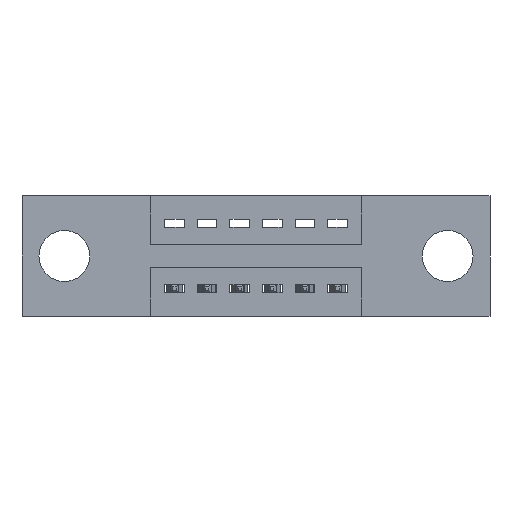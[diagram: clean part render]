
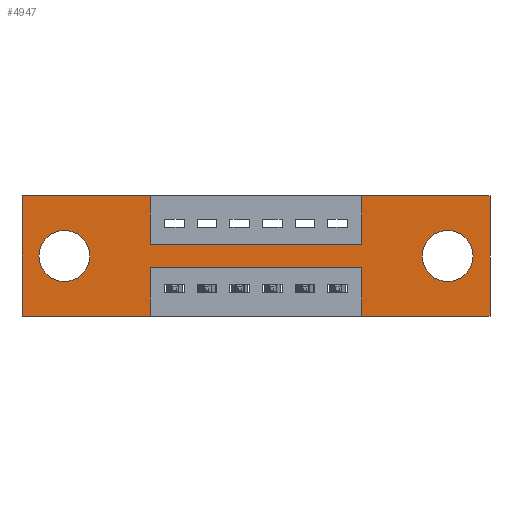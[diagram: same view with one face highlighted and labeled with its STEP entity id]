
A CAD part, front view. The second image highlights one B-rep face of the part: STEP entity #4947.
In plain terms, the highlighted planar face has unit normal (0, -1, 0).
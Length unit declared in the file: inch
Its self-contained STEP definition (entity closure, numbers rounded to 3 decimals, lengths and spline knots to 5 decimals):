
#31 = ORIENTED_EDGE ( 'NONE', *, *, #5997, .F. ) ;
#70 = ORIENTED_EDGE ( 'NONE', *, *, #4666, .F. ) ;
#135 = VECTOR ( 'NONE', #2816, 39.37008 ) ;
#189 = DIRECTION ( 'NONE',  ( 0., 0., -1. ) ) ;
#243 = FACE_BOUND ( 'NONE', #8866, .T. ) ;
#315 = DIRECTION ( 'NONE',  ( 0., 1., 0. ) ) ;
#382 = CARTESIAN_POINT ( 'NONE',  ( 0.13, 0., -0.185 ) ) ;
#444 = AXIS2_PLACEMENT_3D ( 'NONE', #957, #8113, #189 ) ;
#468 = PLANE ( 'NONE',  #444 ) ;
#481 = LINE ( 'NONE', #1972, #6786 ) ;
#488 = CARTESIAN_POINT ( 'NONE',  ( 0.13, 0., -0.263 ) ) ;
#525 = DIRECTION ( 'NONE',  ( 1., 0., 0. ) ) ;
#559 = ORIENTED_EDGE ( 'NONE', *, *, #8038, .F. ) ;
#597 = ORIENTED_EDGE ( 'NONE', *, *, #9324, .F. ) ;
#759 = CARTESIAN_POINT ( 'NONE',  ( 0., 0., 0. ) ) ;
#957 = CARTESIAN_POINT ( 'NONE',  ( 0., 0., -0.37 ) ) ;
#1007 = CARTESIAN_POINT ( 'NONE',  ( 1.0425, 0., 0. ) ) ;
#1058 = VECTOR ( 'NONE', #4355, 39.37008 ) ;
#1109 = CARTESIAN_POINT ( 'NONE',  ( 1.305, 0., -0.263 ) ) ;
#1238 = FACE_BOUND ( 'NONE', #2692, .T. ) ;
#1256 = LINE ( 'NONE', #2137, #6365 ) ;
#1540 = CARTESIAN_POINT ( 'NONE',  ( 0., 0., -0.37 ) ) ;
#1597 = LINE ( 'NONE', #5017, #8882 ) ;
#1707 = VECTOR ( 'NONE', #7568, 39.37008 ) ;
#1757 = EDGE_CURVE ( 'NONE', #7912, #8711, #2393, .T. ) ;
#1902 = CARTESIAN_POINT ( 'NONE',  ( 1.0425, 0., -0.15 ) ) ;
#1972 = CARTESIAN_POINT ( 'NONE',  ( 1.0425, 0., -0.37 ) ) ;
#2090 = EDGE_CURVE ( 'NONE', #6456, #3325, #1597, .T. ) ;
#2092 = CARTESIAN_POINT ( 'NONE',  ( 0.3925, 0., -0.37 ) ) ;
#2137 = CARTESIAN_POINT ( 'NONE',  ( 0., 0., -0.37 ) ) ;
#2390 = EDGE_CURVE ( 'NONE', #7609, #6907, #2963, .T. ) ;
#2393 = LINE ( 'NONE', #4608, #3685 ) ;
#2415 = VERTEX_POINT ( 'NONE', #1109 ) ;
#2526 = LINE ( 'NONE', #7887, #1058 ) ;
#2591 = ORIENTED_EDGE ( 'NONE', *, *, #2090, .F. ) ;
#2649 = EDGE_CURVE ( 'NONE', #6349, #5750, #8670, .T. ) ;
#2692 = EDGE_LOOP ( 'NONE', ( #4839, #3996 ) ) ;
#2729 = EDGE_CURVE ( 'NONE', #6116, #4589, #2526, .T. ) ;
#2816 = DIRECTION ( 'NONE',  ( 0., 0., -1. ) ) ;
#2919 = DIRECTION ( 'NONE',  ( -1., 0., 0. ) ) ;
#2963 = CIRCLE ( 'NONE', #6877, 0.078 ) ;
#3007 = LINE ( 'NONE', #759, #8000 ) ;
#3280 = DIRECTION ( 'NONE',  ( 0., 0., 1. ) ) ;
#3325 = VERTEX_POINT ( 'NONE', #4155 ) ;
#3331 = DIRECTION ( 'NONE',  ( 0., 0., -1. ) ) ;
#3412 = FACE_OUTER_BOUND ( 'NONE', #8729, .T. ) ;
#3461 = CARTESIAN_POINT ( 'NONE',  ( 0.13, 0., -0.185 ) ) ;
#3479 = CARTESIAN_POINT ( 'NONE',  ( 0.3925, 0., 0. ) ) ;
#3500 = EDGE_CURVE ( 'NONE', #8711, #6456, #1256, .T. ) ;
#3652 = VERTEX_POINT ( 'NONE', #3479 ) ;
#3685 = VECTOR ( 'NONE', #8938, 39.37008 ) ;
#3763 = LINE ( 'NONE', #7187, #135 ) ;
#3901 = VERTEX_POINT ( 'NONE', #1902 ) ;
#3996 = ORIENTED_EDGE ( 'NONE', *, *, #9260, .T. ) ;
#4106 = CIRCLE ( 'NONE', #6196, 0.078 ) ;
#4155 = CARTESIAN_POINT ( 'NONE',  ( 0., 0., 0. ) ) ;
#4355 = DIRECTION ( 'NONE',  ( -1., 0., 0. ) ) ;
#4549 = EDGE_CURVE ( 'NONE', #4589, #5044, #481, .T. ) ;
#4589 = VERTEX_POINT ( 'NONE', #5120 ) ;
#4608 = CARTESIAN_POINT ( 'NONE',  ( 0.3925, 0., -0.37 ) ) ;
#4666 = EDGE_CURVE ( 'NONE', #3901, #6349, #6443, .T. ) ;
#4797 = CARTESIAN_POINT ( 'NONE',  ( 1.435, 0., 0. ) ) ;
#4839 = ORIENTED_EDGE ( 'NONE', *, *, #5919, .T. ) ;
#4859 = EDGE_CURVE ( 'NONE', #6907, #7609, #7142, .T. ) ;
#4899 = CARTESIAN_POINT ( 'NONE',  ( 0., 0., 0. ) ) ;
#4905 = ORIENTED_EDGE ( 'NONE', *, *, #1757, .F. ) ;
#4947 = ADVANCED_FACE ( 'NONE', ( #1238, #243, #3412 ), #468, .T. ) ;
#4987 = ORIENTED_EDGE ( 'NONE', *, *, #4549, .F. ) ;
#5003 = ORIENTED_EDGE ( 'NONE', *, *, #4859, .T. ) ;
#5017 = CARTESIAN_POINT ( 'NONE',  ( 0., 0., 0. ) ) ;
#5033 = ORIENTED_EDGE ( 'NONE', *, *, #5449, .F. ) ;
#5044 = VERTEX_POINT ( 'NONE', #5214 ) ;
#5120 = CARTESIAN_POINT ( 'NONE',  ( 1.0425, 0., -0.37 ) ) ;
#5136 = VECTOR ( 'NONE', #9200, 39.37008 ) ;
#5214 = CARTESIAN_POINT ( 'NONE',  ( 1.0425, 0., -0.22 ) ) ;
#5418 = CARTESIAN_POINT ( 'NONE',  ( 1.0425, 0., 0. ) ) ;
#5449 = EDGE_CURVE ( 'NONE', #3652, #5659, #3763, .T. ) ;
#5659 = VERTEX_POINT ( 'NONE', #8985 ) ;
#5750 = VERTEX_POINT ( 'NONE', #4797 ) ;
#5781 = AXIS2_PLACEMENT_3D ( 'NONE', #3461, #315, #8045 ) ;
#5795 = LINE ( 'NONE', #6350, #5136 ) ;
#5919 = EDGE_CURVE ( 'NONE', #6149, #2415, #4106, .T. ) ;
#5944 = CARTESIAN_POINT ( 'NONE',  ( 0.3925, 0., -0.22 ) ) ;
#5997 = EDGE_CURVE ( 'NONE', #5750, #6116, #8730, .T. ) ;
#6029 = ORIENTED_EDGE ( 'NONE', *, *, #2649, .F. ) ;
#6032 = EDGE_CURVE ( 'NONE', #5044, #7912, #5795, .T. ) ;
#6037 = CIRCLE ( 'NONE', #6164, 0.078 ) ;
#6116 = VERTEX_POINT ( 'NONE', #7878 ) ;
#6131 = VECTOR ( 'NONE', #6669, 39.37008 ) ;
#6149 = VERTEX_POINT ( 'NONE', #9357 ) ;
#6164 = AXIS2_PLACEMENT_3D ( 'NONE', #8777, #6601, #7350 ) ;
#6196 = AXIS2_PLACEMENT_3D ( 'NONE', #7641, #8290, #3331 ) ;
#6197 = DIRECTION ( 'NONE',  ( 0., 1., 0. ) ) ;
#6349 = VERTEX_POINT ( 'NONE', #1007 ) ;
#6350 = CARTESIAN_POINT ( 'NONE',  ( 0.3925, 0., -0.22 ) ) ;
#6353 = DIRECTION ( 'NONE',  ( 0., 0., 1. ) ) ;
#6365 = VECTOR ( 'NONE', #2919, 39.37008 ) ;
#6443 = LINE ( 'NONE', #5418, #6131 ) ;
#6456 = VERTEX_POINT ( 'NONE', #1540 ) ;
#6601 = DIRECTION ( 'NONE',  ( 0., 1., 0. ) ) ;
#6669 = DIRECTION ( 'NONE',  ( 0., 0., 1. ) ) ;
#6767 = VECTOR ( 'NONE', #7057, 39.37008 ) ;
#6786 = VECTOR ( 'NONE', #6353, 39.37008 ) ;
#6877 = AXIS2_PLACEMENT_3D ( 'NONE', #382, #6197, #3280 ) ;
#6907 = VERTEX_POINT ( 'NONE', #488 ) ;
#6953 = CARTESIAN_POINT ( 'NONE',  ( 0.3925, 0., -0.15 ) ) ;
#7057 = DIRECTION ( 'NONE',  ( 0., 0., -1. ) ) ;
#7142 = CIRCLE ( 'NONE', #5781, 0.078 ) ;
#7187 = CARTESIAN_POINT ( 'NONE',  ( 0.3925, 0., 0. ) ) ;
#7239 = DIRECTION ( 'NONE',  ( 0., 0., 1. ) ) ;
#7350 = DIRECTION ( 'NONE',  ( 0., 0., -1. ) ) ;
#7480 = LINE ( 'NONE', #6953, #1707 ) ;
#7568 = DIRECTION ( 'NONE',  ( 1., 0., 0. ) ) ;
#7588 = CARTESIAN_POINT ( 'NONE',  ( 0.13, 0., -0.107 ) ) ;
#7609 = VERTEX_POINT ( 'NONE', #7588 ) ;
#7641 = CARTESIAN_POINT ( 'NONE',  ( 1.305, 0., -0.185 ) ) ;
#7867 = VECTOR ( 'NONE', #525, 39.37008 ) ;
#7878 = CARTESIAN_POINT ( 'NONE',  ( 1.435, 0., -0.37 ) ) ;
#7887 = CARTESIAN_POINT ( 'NONE',  ( 0., 0., -0.37 ) ) ;
#7910 = DIRECTION ( 'NONE',  ( 1., 0., 0. ) ) ;
#7912 = VERTEX_POINT ( 'NONE', #5944 ) ;
#7913 = ORIENTED_EDGE ( 'NONE', *, *, #6032, .F. ) ;
#8000 = VECTOR ( 'NONE', #7910, 39.37008 ) ;
#8038 = EDGE_CURVE ( 'NONE', #3325, #3652, #3007, .T. ) ;
#8045 = DIRECTION ( 'NONE',  ( 0., 0., 1. ) ) ;
#8113 = DIRECTION ( 'NONE',  ( 0., -1., 0. ) ) ;
#8161 = ORIENTED_EDGE ( 'NONE', *, *, #2390, .T. ) ;
#8290 = DIRECTION ( 'NONE',  ( 0., 1., 0. ) ) ;
#8670 = LINE ( 'NONE', #4899, #7867 ) ;
#8711 = VERTEX_POINT ( 'NONE', #2092 ) ;
#8729 = EDGE_LOOP ( 'NONE', ( #4905, #7913, #4987, #8990, #31, #6029, #70, #597, #5033, #559, #2591, #9271 ) ) ;
#8730 = LINE ( 'NONE', #9292, #6767 ) ;
#8777 = CARTESIAN_POINT ( 'NONE',  ( 1.305, 0., -0.185 ) ) ;
#8866 = EDGE_LOOP ( 'NONE', ( #8161, #5003 ) ) ;
#8882 = VECTOR ( 'NONE', #7239, 39.37008 ) ;
#8938 = DIRECTION ( 'NONE',  ( 0., 0., -1. ) ) ;
#8985 = CARTESIAN_POINT ( 'NONE',  ( 0.3925, 0., -0.15 ) ) ;
#8990 = ORIENTED_EDGE ( 'NONE', *, *, #2729, .F. ) ;
#9200 = DIRECTION ( 'NONE',  ( -1., 0., 0. ) ) ;
#9260 = EDGE_CURVE ( 'NONE', #2415, #6149, #6037, .T. ) ;
#9271 = ORIENTED_EDGE ( 'NONE', *, *, #3500, .F. ) ;
#9292 = CARTESIAN_POINT ( 'NONE',  ( 1.435, 0., 0. ) ) ;
#9324 = EDGE_CURVE ( 'NONE', #5659, #3901, #7480, .T. ) ;
#9357 = CARTESIAN_POINT ( 'NONE',  ( 1.305, 0., -0.107 ) ) ;
